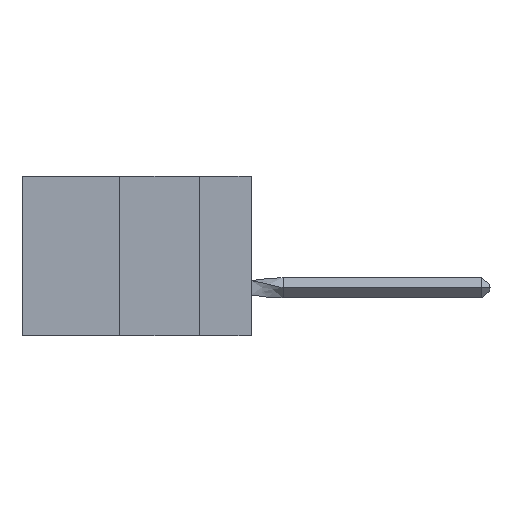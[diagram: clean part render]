
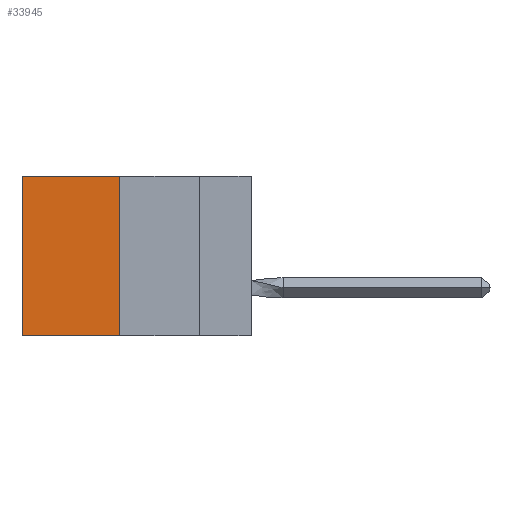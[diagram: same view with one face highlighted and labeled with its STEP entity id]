
A CAD part, left-side view. The second image highlights one B-rep face of the part: STEP entity #33945.
In plain terms, the highlighted planar face has unit normal (-1, 0, 0).
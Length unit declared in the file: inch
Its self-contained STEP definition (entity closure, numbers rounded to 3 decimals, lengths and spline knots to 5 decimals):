
#198 = DIRECTION ( 'NONE',  ( 0., 1., 0. ) ) ;
#606 = VECTOR ( 'NONE', #198, 39.37008 ) ;
#753 = CARTESIAN_POINT ( 'NONE',  ( 0.305, 0.413, -0.5 ) ) ;
#1435 = VERTEX_POINT ( 'NONE', #9111 ) ;
#2158 = VECTOR ( 'NONE', #14741, 39.37008 ) ;
#2327 = VERTEX_POINT ( 'NONE', #34842 ) ;
#2511 = ORIENTED_EDGE ( 'NONE', *, *, #36212, .T. ) ;
#3160 = LINE ( 'NONE', #4099, #10312 ) ;
#3560 = DIRECTION ( 'NONE',  ( 1., 0., 0. ) ) ;
#4099 = CARTESIAN_POINT ( 'NONE',  ( 0.305, 0.413, 0. ) ) ;
#8905 = LINE ( 'NONE', #32888, #2158 ) ;
#9111 = CARTESIAN_POINT ( 'NONE',  ( 0.305, 0.413, -0.5 ) ) ;
#9577 = LINE ( 'NONE', #15851, #34030 ) ;
#10272 = FACE_OUTER_BOUND ( 'NONE', #20505, .T. ) ;
#10312 = VECTOR ( 'NONE', #28603, 39.37008 ) ;
#11117 = VERTEX_POINT ( 'NONE', #21964 ) ;
#13387 = EDGE_CURVE ( 'NONE', #1435, #2327, #24181, .T. ) ;
#14686 = CARTESIAN_POINT ( 'NONE',  ( 0.305, 0.413, 0. ) ) ;
#14741 = DIRECTION ( 'NONE',  ( 0., 0., -1. ) ) ;
#15307 = CARTESIAN_POINT ( 'NONE',  ( 0.305, 0.413, -0.5 ) ) ;
#15675 = EDGE_CURVE ( 'NONE', #26083, #1435, #8905, .T. ) ;
#15851 = CARTESIAN_POINT ( 'NONE',  ( 0.305, 0.72, -0.5 ) ) ;
#18505 = PLANE ( 'NONE',  #31324 ) ;
#20505 = EDGE_LOOP ( 'NONE', ( #2511, #32675, #22831, #24616 ) ) ;
#21964 = CARTESIAN_POINT ( 'NONE',  ( 0.305, 0.72, 0. ) ) ;
#22831 = ORIENTED_EDGE ( 'NONE', *, *, #15675, .F. ) ;
#24181 = LINE ( 'NONE', #753, #606 ) ;
#24616 = ORIENTED_EDGE ( 'NONE', *, *, #33182, .T. ) ;
#24647 = DIRECTION ( 'NONE',  ( 0., 0., -1. ) ) ;
#26083 = VERTEX_POINT ( 'NONE', #14686 ) ;
#28603 = DIRECTION ( 'NONE',  ( 0., 1., 0. ) ) ;
#31324 = AXIS2_PLACEMENT_3D ( 'NONE', #15307, #3560, #24647 ) ;
#32675 = ORIENTED_EDGE ( 'NONE', *, *, #13387, .F. ) ;
#32888 = CARTESIAN_POINT ( 'NONE',  ( 0.305, 0.413, -0.5 ) ) ;
#33182 = EDGE_CURVE ( 'NONE', #26083, #11117, #3160, .T. ) ;
#33945 = ADVANCED_FACE ( 'NONE', ( #10272 ), #18505, .F. ) ;
#34030 = VECTOR ( 'NONE', #37580, 39.37008 ) ;
#34842 = CARTESIAN_POINT ( 'NONE',  ( 0.305, 0.72, -0.5 ) ) ;
#36212 = EDGE_CURVE ( 'NONE', #11117, #2327, #9577, .T. ) ;
#37580 = DIRECTION ( 'NONE',  ( 0., 0., -1. ) ) ;
